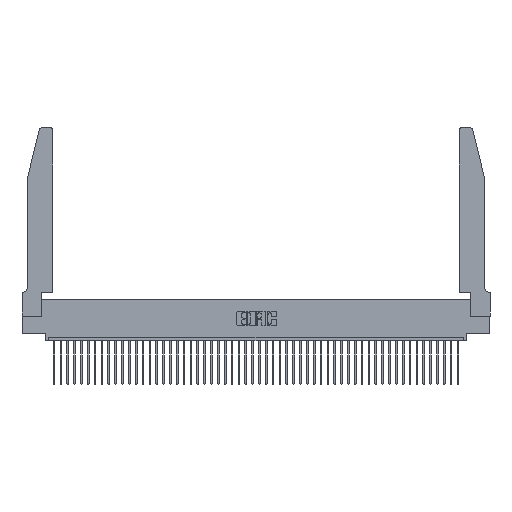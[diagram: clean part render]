
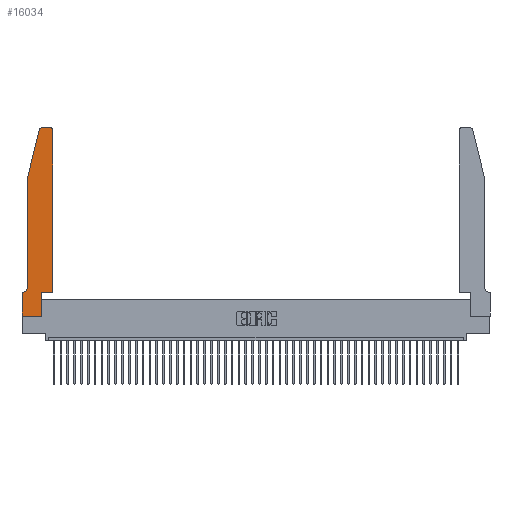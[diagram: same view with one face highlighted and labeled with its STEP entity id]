
A CAD part, top view. The second image highlights one B-rep face of the part: STEP entity #16034.
In plain terms, the highlighted planar face has unit normal (0, 0, 1).
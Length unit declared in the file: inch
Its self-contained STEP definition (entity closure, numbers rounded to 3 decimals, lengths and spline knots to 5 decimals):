
#629 = ORIENTED_EDGE ( 'NONE', *, *, #5010, .T. ) ;
#755 = ORIENTED_EDGE ( 'NONE', *, *, #10924, .T. ) ;
#757 = CARTESIAN_POINT ( 'NONE',  ( 0.0755, 0.35, 0.37 ) ) ;
#793 = CARTESIAN_POINT ( 'NONE',  ( 0.2865, 0., 0.37 ) ) ;
#1958 = DIRECTION ( 'NONE',  ( -1., 0., 0. ) ) ;
#2949 = LINE ( 'NONE', #23653, #28905 ) ;
#3127 = AXIS2_PLACEMENT_3D ( 'NONE', #26458, #8218, #19646 ) ;
#3763 = LINE ( 'NONE', #38596, #22773 ) ;
#3926 = VECTOR ( 'NONE', #33839, 39.37008 ) ;
#3927 = VERTEX_POINT ( 'NONE', #21238 ) ;
#4165 = DIRECTION ( 'NONE',  ( 1., 0., 0. ) ) ;
#5010 = EDGE_CURVE ( 'NONE', #20834, #44862, #13773, .T. ) ;
#5202 = CARTESIAN_POINT ( 'NONE',  ( 0.284, 2.72, 0.37 ) ) ;
#5929 = ORIENTED_EDGE ( 'NONE', *, *, #14395, .T. ) ;
#6004 = VERTEX_POINT ( 'NONE', #29841 ) ;
#7367 = ORIENTED_EDGE ( 'NONE', *, *, #40175, .T. ) ;
#7407 = CARTESIAN_POINT ( 'NONE',  ( 0., 0., 0.37 ) ) ;
#8218 = DIRECTION ( 'NONE',  ( 0., 0., 1. ) ) ;
#9058 = CARTESIAN_POINT ( 'NONE',  ( 0.4505, 2.72, 0.37 ) ) ;
#9254 = VECTOR ( 'NONE', #11536, 39.37008 ) ;
#9590 = DIRECTION ( 'NONE',  ( 0., 0., 1. ) ) ;
#10071 = CARTESIAN_POINT ( 'NONE',  ( 0.4205, 2.72, 0.37 ) ) ;
#10924 = EDGE_CURVE ( 'NONE', #34696, #18092, #32749, .T. ) ;
#11536 = DIRECTION ( 'NONE',  ( -1., 0., 0. ) ) ;
#12345 = ORIENTED_EDGE ( 'NONE', *, *, #14309, .T. ) ;
#12498 = CARTESIAN_POINT ( 'NONE',  ( 0.4505, 0.35, 0.37 ) ) ;
#12742 = LINE ( 'NONE', #33496, #31753 ) ;
#13361 = VECTOR ( 'NONE', #4165, 39.37008 ) ;
#13773 = CIRCLE ( 'NONE', #42841, 0.07 ) ;
#13799 = CARTESIAN_POINT ( 'NONE',  ( 0.0755, 2., 0.37 ) ) ;
#14309 = EDGE_CURVE ( 'NONE', #25056, #34696, #12742, .T. ) ;
#14395 = EDGE_CURVE ( 'NONE', #35124, #20489, #2949, .T. ) ;
#15753 = CARTESIAN_POINT ( 'NONE',  ( 0.0755, 2., 0.37 ) ) ;
#16034 = ADVANCED_FACE ( 'NONE', ( #32217 ), #45177, .T. ) ;
#16209 = CARTESIAN_POINT ( 'NONE',  ( 0., 0., 0.37 ) ) ;
#16537 = DIRECTION ( 'NONE',  ( -0.239, -0.971, 0. ) ) ;
#16619 = DIRECTION ( 'NONE',  ( 1., 0., 0. ) ) ;
#16737 = EDGE_CURVE ( 'NONE', #26739, #20834, #19213, .T. ) ;
#17932 = EDGE_CURVE ( 'NONE', #20489, #35117, #42688, .T. ) ;
#18092 = VERTEX_POINT ( 'NONE', #41307 ) ;
#18429 = CARTESIAN_POINT ( 'NONE',  ( 0.2865, 0.35, 0.37 ) ) ;
#18568 = CARTESIAN_POINT ( 'NONE',  ( 0.2865, 0.35, 0.37 ) ) ;
#18651 = CARTESIAN_POINT ( 'NONE',  ( 0., 0.35, 0.37 ) ) ;
#18887 = VECTOR ( 'NONE', #41601, 39.37008 ) ;
#19213 = LINE ( 'NONE', #15753, #26724 ) ;
#19646 = DIRECTION ( 'NONE',  ( 1., 0., 0. ) ) ;
#19715 = EDGE_CURVE ( 'NONE', #44325, #25056, #33312, .T. ) ;
#19804 = DIRECTION ( 'NONE',  ( 0., -1., 0. ) ) ;
#20489 = VERTEX_POINT ( 'NONE', #16209 ) ;
#20834 = VERTEX_POINT ( 'NONE', #22779 ) ;
#20934 = EDGE_CURVE ( 'NONE', #35117, #44325, #42932, .T. ) ;
#21238 = CARTESIAN_POINT ( 'NONE',  ( 0.25487, 2.72718, 0.37 ) ) ;
#22751 = DIRECTION ( 'NONE',  ( 0., 1., 0. ) ) ;
#22773 = VECTOR ( 'NONE', #16537, 39.37008 ) ;
#22779 = CARTESIAN_POINT ( 'NONE',  ( 0.0755, 0.42, 0.37 ) ) ;
#23508 = CARTESIAN_POINT ( 'NONE',  ( 0.4505, 0.35, 0.37 ) ) ;
#23653 = CARTESIAN_POINT ( 'NONE',  ( 0., 0., 0.37 ) ) ;
#24391 = EDGE_CURVE ( 'NONE', #18092, #6004, #32718, .T. ) ;
#25056 = VERTEX_POINT ( 'NONE', #23508 ) ;
#25430 = DIRECTION ( 'NONE',  ( 0., -1., 0. ) ) ;
#26458 = CARTESIAN_POINT ( 'NONE',  ( 0., 0.35, 0.37 ) ) ;
#26724 = VECTOR ( 'NONE', #19804, 39.37008 ) ;
#26739 = VERTEX_POINT ( 'NONE', #13799 ) ;
#27257 = CARTESIAN_POINT ( 'NONE',  ( 0.0055, 0.42, 0.37 ) ) ;
#27998 = AXIS2_PLACEMENT_3D ( 'NONE', #5202, #31447, #16619 ) ;
#28746 = ORIENTED_EDGE ( 'NONE', *, *, #20934, .T. ) ;
#28905 = VECTOR ( 'NONE', #25430, 39.37008 ) ;
#28916 = EDGE_CURVE ( 'NONE', #44862, #35124, #30581, .T. ) ;
#29841 = CARTESIAN_POINT ( 'NONE',  ( 0.284, 2.75, 0.37 ) ) ;
#30581 = LINE ( 'NONE', #757, #9254 ) ;
#31447 = DIRECTION ( 'NONE',  ( 0., 0., 1. ) ) ;
#31753 = VECTOR ( 'NONE', #34127, 39.37008 ) ;
#31787 = ORIENTED_EDGE ( 'NONE', *, *, #45882, .T. ) ;
#32217 = FACE_OUTER_BOUND ( 'NONE', #45651, .T. ) ;
#32493 = ORIENTED_EDGE ( 'NONE', *, *, #28916, .T. ) ;
#32718 = LINE ( 'NONE', #45027, #3926 ) ;
#32749 = CIRCLE ( 'NONE', #41226, 0.03 ) ;
#32834 = ORIENTED_EDGE ( 'NONE', *, *, #16737, .T. ) ;
#33312 = LINE ( 'NONE', #12498, #18887 ) ;
#33496 = CARTESIAN_POINT ( 'NONE',  ( 0.4505, 0.35, 0.37 ) ) ;
#33741 = VECTOR ( 'NONE', #22751, 39.37008 ) ;
#33839 = DIRECTION ( 'NONE',  ( -1., 0., 0. ) ) ;
#34127 = DIRECTION ( 'NONE',  ( 0., 1., 0. ) ) ;
#34696 = VERTEX_POINT ( 'NONE', #9058 ) ;
#35117 = VERTEX_POINT ( 'NONE', #793 ) ;
#35124 = VERTEX_POINT ( 'NONE', #18651 ) ;
#38596 = CARTESIAN_POINT ( 'NONE',  ( 0.0755, 2., 0.37 ) ) ;
#40175 = EDGE_CURVE ( 'NONE', #6004, #3927, #40195, .T. ) ;
#40185 = ORIENTED_EDGE ( 'NONE', *, *, #24391, .T. ) ;
#40195 = CIRCLE ( 'NONE', #27998, 0.03 ) ;
#40900 = CARTESIAN_POINT ( 'NONE',  ( 0.0055, 0.35, 0.37 ) ) ;
#41226 = AXIS2_PLACEMENT_3D ( 'NONE', #10071, #9590, #46398 ) ;
#41307 = CARTESIAN_POINT ( 'NONE',  ( 0.4205, 2.75, 0.37 ) ) ;
#41601 = DIRECTION ( 'NONE',  ( 1., 0., 0. ) ) ;
#42688 = LINE ( 'NONE', #7407, #13361 ) ;
#42841 = AXIS2_PLACEMENT_3D ( 'NONE', #27257, #45522, #1958 ) ;
#42932 = LINE ( 'NONE', #18568, #33741 ) ;
#43313 = ORIENTED_EDGE ( 'NONE', *, *, #19715, .T. ) ;
#44325 = VERTEX_POINT ( 'NONE', #18429 ) ;
#44862 = VERTEX_POINT ( 'NONE', #40900 ) ;
#45027 = CARTESIAN_POINT ( 'NONE',  ( 0.2605, 2.75, 0.37 ) ) ;
#45177 = PLANE ( 'NONE',  #3127 ) ;
#45522 = DIRECTION ( 'NONE',  ( 0., 0., -1. ) ) ;
#45651 = EDGE_LOOP ( 'NONE', ( #40185, #7367, #31787, #32834, #629, #32493, #5929, #46257, #28746, #43313, #12345, #755 ) ) ;
#45882 = EDGE_CURVE ( 'NONE', #3927, #26739, #3763, .T. ) ;
#46257 = ORIENTED_EDGE ( 'NONE', *, *, #17932, .T. ) ;
#46398 = DIRECTION ( 'NONE',  ( 1., 0., 0. ) ) ;
